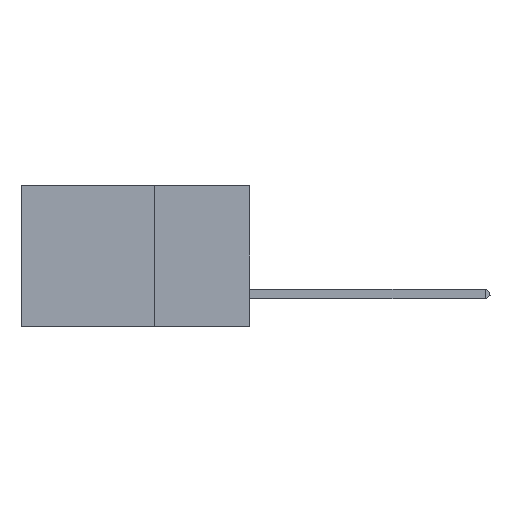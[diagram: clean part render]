
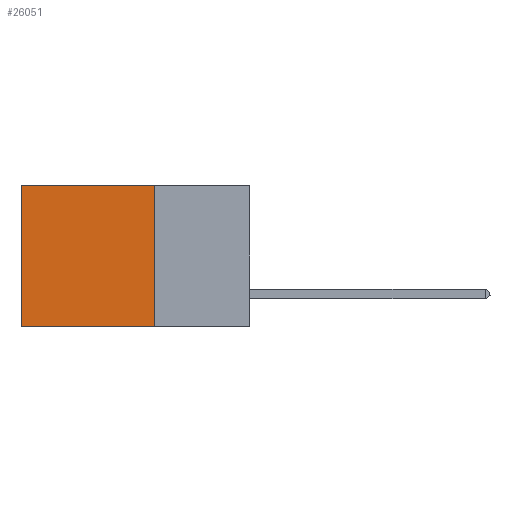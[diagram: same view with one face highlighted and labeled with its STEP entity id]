
A CAD part, left-side view. The second image highlights one B-rep face of the part: STEP entity #26051.
In plain terms, the highlighted planar face has unit normal (-1, 0, 0).
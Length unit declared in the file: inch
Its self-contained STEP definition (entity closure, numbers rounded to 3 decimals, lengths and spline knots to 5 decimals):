
#169 = EDGE_CURVE ( 'NONE', #30613, #12302, #29746, .T. ) ;
#1220 = EDGE_CURVE ( 'NONE', #25964, #30613, #7667, .T. ) ;
#2430 = EDGE_CURVE ( 'NONE', #25964, #40744, #27952, .T. ) ;
#3569 = VECTOR ( 'NONE', #6595, 39.37008 ) ;
#4979 = CARTESIAN_POINT ( 'NONE',  ( 0.2875, 0.25, 0. ) ) ;
#5339 = CARTESIAN_POINT ( 'NONE',  ( 0.2875, 0.25, 0. ) ) ;
#5605 = FACE_OUTER_BOUND ( 'NONE', #11041, .T. ) ;
#6595 = DIRECTION ( 'NONE',  ( 0., 0., -1. ) ) ;
#7667 = LINE ( 'NONE', #4979, #33299 ) ;
#10888 = ORIENTED_EDGE ( 'NONE', *, *, #169, .F. ) ;
#11041 = EDGE_LOOP ( 'NONE', ( #23558, #10888, #30410, #17724 ) ) ;
#12302 = VERTEX_POINT ( 'NONE', #34701 ) ;
#12634 = PLANE ( 'NONE',  #41125 ) ;
#12917 = DIRECTION ( 'NONE',  ( 0., 0., -1. ) ) ;
#13516 = CARTESIAN_POINT ( 'NONE',  ( 0.2875, 0.25, -0.37 ) ) ;
#15153 = CARTESIAN_POINT ( 'NONE',  ( 0.2875, 0.6, 0. ) ) ;
#17724 = ORIENTED_EDGE ( 'NONE', *, *, #2430, .T. ) ;
#19277 = VECTOR ( 'NONE', #41031, 39.37008 ) ;
#19580 = DIRECTION ( 'NONE',  ( 0., 0., -1. ) ) ;
#23558 = ORIENTED_EDGE ( 'NONE', *, *, #32243, .T. ) ;
#25964 = VERTEX_POINT ( 'NONE', #5339 ) ;
#26051 = ADVANCED_FACE ( 'NONE', ( #5605 ), #12634, .F. ) ;
#26215 = DIRECTION ( 'NONE',  ( 1., 0., 0. ) ) ;
#27952 = LINE ( 'NONE', #29955, #42085 ) ;
#29746 = LINE ( 'NONE', #13516, #19277 ) ;
#29955 = CARTESIAN_POINT ( 'NONE',  ( 0.2875, 0.25, 0. ) ) ;
#30410 = ORIENTED_EDGE ( 'NONE', *, *, #1220, .F. ) ;
#30530 = DIRECTION ( 'NONE',  ( 0., 1., 0. ) ) ;
#30613 = VERTEX_POINT ( 'NONE', #43061 ) ;
#32243 = EDGE_CURVE ( 'NONE', #40744, #12302, #41756, .T. ) ;
#33060 = CARTESIAN_POINT ( 'NONE',  ( 0.2875, 0.6, 0. ) ) ;
#33299 = VECTOR ( 'NONE', #19580, 39.37008 ) ;
#34701 = CARTESIAN_POINT ( 'NONE',  ( 0.2875, 0.6, -0.37 ) ) ;
#36186 = CARTESIAN_POINT ( 'NONE',  ( 0.2875, 0.25, 0. ) ) ;
#40744 = VERTEX_POINT ( 'NONE', #15153 ) ;
#41031 = DIRECTION ( 'NONE',  ( 0., 1., 0. ) ) ;
#41125 = AXIS2_PLACEMENT_3D ( 'NONE', #36186, #26215, #12917 ) ;
#41756 = LINE ( 'NONE', #33060, #3569 ) ;
#42085 = VECTOR ( 'NONE', #30530, 39.37008 ) ;
#43061 = CARTESIAN_POINT ( 'NONE',  ( 0.2875, 0.25, -0.37 ) ) ;
